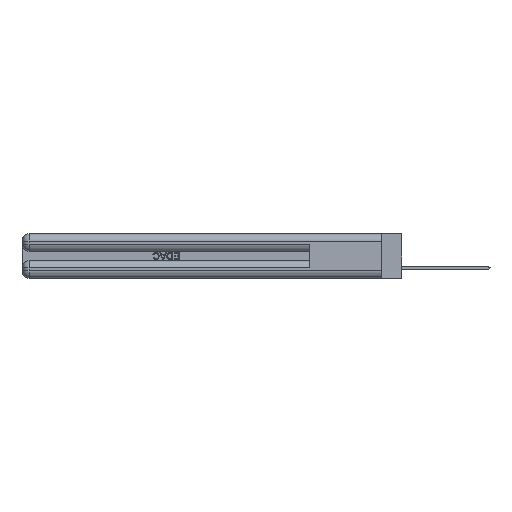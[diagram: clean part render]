
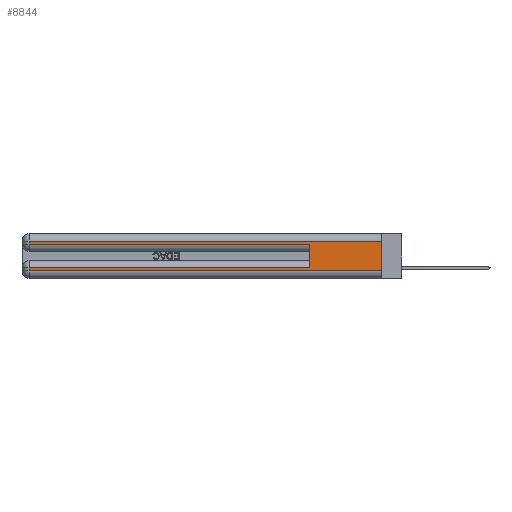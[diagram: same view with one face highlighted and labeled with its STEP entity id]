
A CAD part, left-side view. The second image highlights one B-rep face of the part: STEP entity #8844.
In plain terms, the highlighted planar face has unit normal (-1, 0, 0).
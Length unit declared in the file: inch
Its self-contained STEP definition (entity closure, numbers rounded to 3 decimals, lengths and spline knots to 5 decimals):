
#1687 = LINE ( 'NONE', #36494, #26624 ) ;
#1781 = EDGE_LOOP ( 'NONE', ( #18350, #3403, #47017, #4090, #30001, #13971, #30976, #34323 ) ) ;
#2565 = VERTEX_POINT ( 'NONE', #33612 ) ;
#3334 = EDGE_CURVE ( 'NONE', #30417, #14938, #24625, .T. ) ;
#3403 = ORIENTED_EDGE ( 'NONE', *, *, #38395, .T. ) ;
#3480 = EDGE_CURVE ( 'NONE', #31500, #47429, #46536, .T. ) ;
#4090 = ORIENTED_EDGE ( 'NONE', *, *, #3334, .T. ) ;
#4223 = VECTOR ( 'NONE', #34754, 39.37008 ) ;
#4274 = VERTEX_POINT ( 'NONE', #25167 ) ;
#5412 = EDGE_CURVE ( 'NONE', #2565, #31500, #41794, .T. ) ;
#7821 = VERTEX_POINT ( 'NONE', #26745 ) ;
#8758 = VECTOR ( 'NONE', #11551, 39.37008 ) ;
#8844 = ADVANCED_FACE ( 'NONE', ( #23518 ), #20232, .F. ) ;
#9351 = CARTESIAN_POINT ( 'NONE',  ( 0., 0.6, 0.085 ) ) ;
#9523 = EDGE_CURVE ( 'NONE', #14031, #14938, #35753, .T. ) ;
#10919 = VECTOR ( 'NONE', #34924, 39.37008 ) ;
#11551 = DIRECTION ( 'NONE',  ( 0., 0., -1. ) ) ;
#12026 = CARTESIAN_POINT ( 'NONE',  ( 0., 0., 0.37 ) ) ;
#13971 = ORIENTED_EDGE ( 'NONE', *, *, #15017, .T. ) ;
#14031 = VERTEX_POINT ( 'NONE', #9351 ) ;
#14097 = CARTESIAN_POINT ( 'NONE',  ( 0., 0., 0.285 ) ) ;
#14938 = VERTEX_POINT ( 'NONE', #21882 ) ;
#15017 = EDGE_CURVE ( 'NONE', #14031, #2565, #46737, .T. ) ;
#15679 = CARTESIAN_POINT ( 'NONE',  ( 0., 0., 0.06 ) ) ;
#15826 = DIRECTION ( 'NONE',  ( 0., 0., -1. ) ) ;
#18350 = ORIENTED_EDGE ( 'NONE', *, *, #20736, .F. ) ;
#19593 = CARTESIAN_POINT ( 'NONE',  ( 0., 0., 0.37 ) ) ;
#19609 = CARTESIAN_POINT ( 'NONE',  ( 0., 2.94, 0.06 ) ) ;
#19869 = CARTESIAN_POINT ( 'NONE',  ( 0., 2.94, 0.285 ) ) ;
#20118 = VECTOR ( 'NONE', #25031, 39.37008 ) ;
#20232 = PLANE ( 'NONE',  #44152 ) ;
#20736 = EDGE_CURVE ( 'NONE', #4274, #47429, #22075, .T. ) ;
#20945 = DIRECTION ( 'NONE',  ( 0., -1., 0. ) ) ;
#21707 = EDGE_CURVE ( 'NONE', #7821, #30417, #1687, .T. ) ;
#21829 = DIRECTION ( 'NONE',  ( 0., 1., 0. ) ) ;
#21882 = CARTESIAN_POINT ( 'NONE',  ( 0., 0.6, 0.285 ) ) ;
#22075 = LINE ( 'NONE', #12026, #8758 ) ;
#23518 = FACE_OUTER_BOUND ( 'NONE', #1781, .T. ) ;
#24625 = LINE ( 'NONE', #14097, #26388 ) ;
#25031 = DIRECTION ( 'NONE',  ( 0., 0., 1. ) ) ;
#25167 = CARTESIAN_POINT ( 'NONE',  ( 0., 0., 0.31 ) ) ;
#25785 = VECTOR ( 'NONE', #33951, 39.37008 ) ;
#26388 = VECTOR ( 'NONE', #20945, 39.37008 ) ;
#26624 = VECTOR ( 'NONE', #44956, 39.37008 ) ;
#26745 = CARTESIAN_POINT ( 'NONE',  ( 0., 2.94, 0.31 ) ) ;
#27578 = CARTESIAN_POINT ( 'NONE',  ( 0., 2.94, 0.37 ) ) ;
#28459 = CARTESIAN_POINT ( 'NONE',  ( 0., 0.6, 0.145 ) ) ;
#28754 = LINE ( 'NONE', #32982, #29309 ) ;
#29309 = VECTOR ( 'NONE', #21829, 39.37008 ) ;
#30001 = ORIENTED_EDGE ( 'NONE', *, *, #9523, .F. ) ;
#30417 = VERTEX_POINT ( 'NONE', #19869 ) ;
#30976 = ORIENTED_EDGE ( 'NONE', *, *, #5412, .T. ) ;
#31500 = VERTEX_POINT ( 'NONE', #19609 ) ;
#32982 = CARTESIAN_POINT ( 'NONE',  ( 0., 0., 0.31 ) ) ;
#33612 = CARTESIAN_POINT ( 'NONE',  ( 0., 2.94, 0.085 ) ) ;
#33951 = DIRECTION ( 'NONE',  ( 0., -1., 0. ) ) ;
#34323 = ORIENTED_EDGE ( 'NONE', *, *, #3480, .T. ) ;
#34414 = DIRECTION ( 'NONE',  ( 1., 0., 0. ) ) ;
#34754 = DIRECTION ( 'NONE',  ( 0., 0., -1. ) ) ;
#34924 = DIRECTION ( 'NONE',  ( 0., 1., 0. ) ) ;
#35371 = CARTESIAN_POINT ( 'NONE',  ( 0., 0., 0.085 ) ) ;
#35753 = LINE ( 'NONE', #28459, #20118 ) ;
#36494 = CARTESIAN_POINT ( 'NONE',  ( 0., 2.94, 0.37 ) ) ;
#38395 = EDGE_CURVE ( 'NONE', #4274, #7821, #28754, .T. ) ;
#41585 = CARTESIAN_POINT ( 'NONE',  ( 0., 0., 0.06 ) ) ;
#41794 = LINE ( 'NONE', #27578, #4223 ) ;
#44152 = AXIS2_PLACEMENT_3D ( 'NONE', #19593, #34414, #15826 ) ;
#44956 = DIRECTION ( 'NONE',  ( 0., 0., -1. ) ) ;
#46536 = LINE ( 'NONE', #15679, #25785 ) ;
#46737 = LINE ( 'NONE', #35371, #10919 ) ;
#47017 = ORIENTED_EDGE ( 'NONE', *, *, #21707, .T. ) ;
#47429 = VERTEX_POINT ( 'NONE', #41585 ) ;
